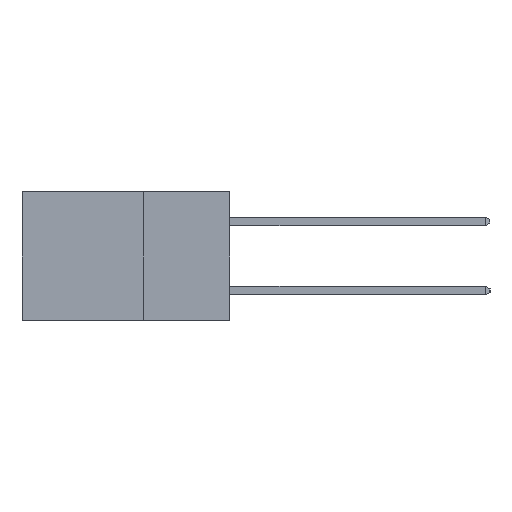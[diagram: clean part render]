
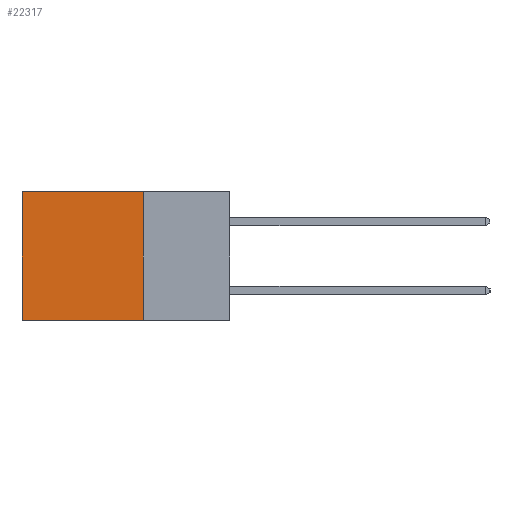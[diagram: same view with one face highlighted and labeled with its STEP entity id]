
A CAD part, left-side view. The second image highlights one B-rep face of the part: STEP entity #22317.
In plain terms, the highlighted planar face has unit normal (-1, 0, 0).
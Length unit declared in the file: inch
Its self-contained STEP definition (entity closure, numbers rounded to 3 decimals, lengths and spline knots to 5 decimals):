
#409 = PLANE ( 'NONE',  #2114 ) ;
#1830 = DIRECTION ( 'NONE',  ( 0., 0., -1. ) ) ;
#2114 = AXIS2_PLACEMENT_3D ( 'NONE', #19244, #15635, #4211 ) ;
#2686 = LINE ( 'NONE', #12243, #12309 ) ;
#3731 = CARTESIAN_POINT ( 'NONE',  ( 0.2615, 0.25, -0.37 ) ) ;
#3956 = CARTESIAN_POINT ( 'NONE',  ( 0.2615, 0.25, -0.37 ) ) ;
#4154 = DIRECTION ( 'NONE',  ( 0., 1., 0. ) ) ;
#4211 = DIRECTION ( 'NONE',  ( 0., 0., -1. ) ) ;
#7523 = CARTESIAN_POINT ( 'NONE',  ( 0.2615, 0.6, -0.37 ) ) ;
#8160 = CARTESIAN_POINT ( 'NONE',  ( 0.2615, 0.6, 0. ) ) ;
#8396 = LINE ( 'NONE', #3731, #22676 ) ;
#11289 = VERTEX_POINT ( 'NONE', #3956 ) ;
#12243 = CARTESIAN_POINT ( 'NONE',  ( 0.2615, 0.25, -0.37 ) ) ;
#12309 = VECTOR ( 'NONE', #14128, 39.37008 ) ;
#13378 = DIRECTION ( 'NONE',  ( 0., 0., -1. ) ) ;
#13947 = ORIENTED_EDGE ( 'NONE', *, *, #21647, .T. ) ;
#14128 = DIRECTION ( 'NONE',  ( 0., 1., 0. ) ) ;
#14768 = ORIENTED_EDGE ( 'NONE', *, *, #15686, .T. ) ;
#15585 = CARTESIAN_POINT ( 'NONE',  ( 0.2615, 0.25, 0. ) ) ;
#15635 = DIRECTION ( 'NONE',  ( 1., 0., 0. ) ) ;
#15686 = EDGE_CURVE ( 'NONE', #22347, #22358, #23678, .T. ) ;
#16039 = VERTEX_POINT ( 'NONE', #18121 ) ;
#17122 = FACE_OUTER_BOUND ( 'NONE', #21786, .T. ) ;
#17556 = CARTESIAN_POINT ( 'NONE',  ( 0.2615, 0.6, -0.37 ) ) ;
#17724 = LINE ( 'NONE', #15585, #18304 ) ;
#18121 = CARTESIAN_POINT ( 'NONE',  ( 0.2615, 0.25, 0. ) ) ;
#18140 = EDGE_CURVE ( 'NONE', #11289, #22358, #2686, .T. ) ;
#18304 = VECTOR ( 'NONE', #4154, 39.37008 ) ;
#18542 = EDGE_CURVE ( 'NONE', #16039, #11289, #8396, .T. ) ;
#18961 = ORIENTED_EDGE ( 'NONE', *, *, #18140, .F. ) ;
#19244 = CARTESIAN_POINT ( 'NONE',  ( 0.2615, 0.25, -0.37 ) ) ;
#19981 = VECTOR ( 'NONE', #1830, 39.37008 ) ;
#21647 = EDGE_CURVE ( 'NONE', #16039, #22347, #17724, .T. ) ;
#21786 = EDGE_LOOP ( 'NONE', ( #14768, #18961, #24131, #13947 ) ) ;
#22317 = ADVANCED_FACE ( 'NONE', ( #17122 ), #409, .F. ) ;
#22347 = VERTEX_POINT ( 'NONE', #8160 ) ;
#22358 = VERTEX_POINT ( 'NONE', #17556 ) ;
#22676 = VECTOR ( 'NONE', #13378, 39.37008 ) ;
#23678 = LINE ( 'NONE', #7523, #19981 ) ;
#24131 = ORIENTED_EDGE ( 'NONE', *, *, #18542, .F. ) ;
